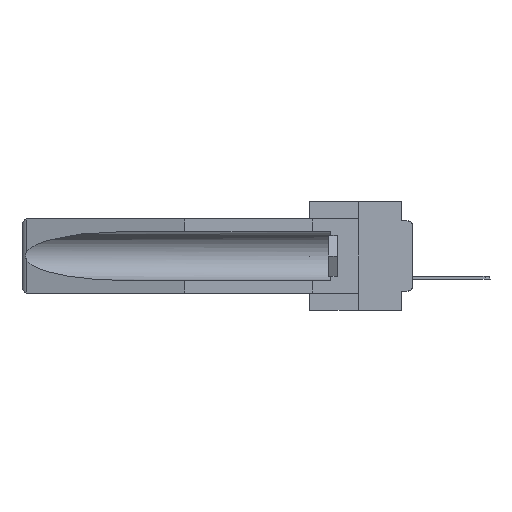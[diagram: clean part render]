
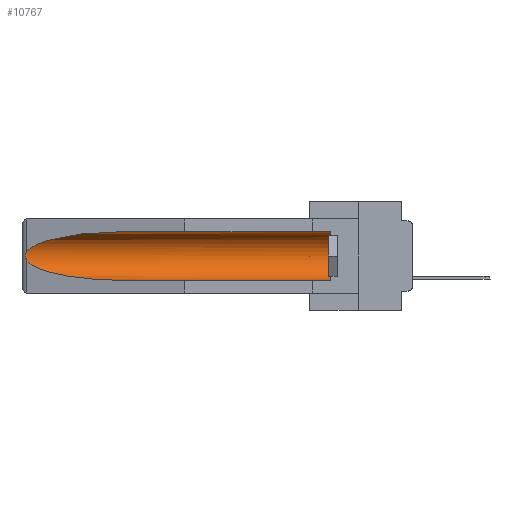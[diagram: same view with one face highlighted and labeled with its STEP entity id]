
A CAD part, left-side view. The second image highlights one B-rep face of the part: STEP entity #10767.
In plain terms, the highlighted cylindrical face has radius 2.857 mm (diameter 5.715 mm), a partial arc.
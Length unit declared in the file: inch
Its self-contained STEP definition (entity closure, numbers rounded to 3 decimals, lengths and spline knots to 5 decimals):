
#96 = ORIENTED_EDGE ( 'NONE', *, *, #34960, .F. ) ;
#110 = CARTESIAN_POINT ( 'NONE',  ( 0.25451, 1.48313, -0.09465 ) ) ;
#827 = CARTESIAN_POINT ( 'NONE',  ( 0.2673, 1.53269, -0.17917 ) ) ;
#1669 = VERTEX_POINT ( 'NONE', #9027 ) ;
#2537 = EDGE_CURVE ( 'NONE', #20760, #1669, #23115, .T. ) ;
#2706 = CARTESIAN_POINT ( 'NONE',  ( 0.155, -0.30754, -0.1715 ) ) ;
#2724 = CARTESIAN_POINT ( 'NONE',  ( 0.21114, 1.30732, -0.284 ) ) ;
#2728 = DIRECTION ( 'NONE',  ( 0., 1., 0. ) ) ;
#4487 = CARTESIAN_POINT ( 'NONE',  ( 0.26655, 1.53094, -0.18657 ) ) ;
#4593 = LINE ( 'NONE', #16008, #13410 ) ;
#5051 = B_SPLINE_CURVE_WITH_KNOTS ( 'NONE', 3,
 ( #12749, #19198, #12609, #27649, #9901, #18641, #827, #4487, #19465, #10458 ),
 .UNSPECIFIED., .F., .F.,
 ( 4, 2, 2, 2, 4 ),
 ( 0., 0.00029, 0.00058, 0.00087, 0.00117 ),
 .UNSPECIFIED. ) ;
#6569 = EDGE_CURVE ( 'NONE', #15668, #6992, #25724, .T. ) ;
#6992 = VERTEX_POINT ( 'NONE', #28050 ) ;
#7362 = CARTESIAN_POINT ( 'NONE',  ( 0.155, -0.30754, -0.059 ) ) ;
#7677 = VERTEX_POINT ( 'NONE', #29914 ) ;
#8663 = DIRECTION ( 'NONE',  ( 0., 0., 1. ) ) ;
#8772 = DIRECTION ( 'NONE',  ( 0., 1., 0. ) ) ;
#8886 = LINE ( 'NONE', #7362, #9338 ) ;
#9027 = CARTESIAN_POINT ( 'NONE',  ( 0.155, 0.126, -0.059 ) ) ;
#9338 = VECTOR ( 'NONE', #2728, 39.37008 ) ;
#9855 = EDGE_CURVE ( 'NONE', #1669, #15668, #8886, .T. ) ;
#9901 = CARTESIAN_POINT ( 'NONE',  ( 0.2675, 1.53308, -0.16763 ) ) ;
#10092 = ORIENTED_EDGE ( 'NONE', *, *, #10368, .T. ) ;
#10368 = EDGE_CURVE ( 'NONE', #7677, #26280, #29241, .T. ) ;
#10458 = CARTESIAN_POINT ( 'NONE',  ( 0.26537, 1.52718, -0.19328 ) ) ;
#10767 = ADVANCED_FACE ( 'NONE', ( #35269 ), #16749, .F. ) ;
#10997 = ORIENTED_EDGE ( 'NONE', *, *, #2537, .T. ) ;
#12609 = CARTESIAN_POINT ( 'NONE',  ( 0.26654, 1.53092, -0.15636 ) ) ;
#12749 = CARTESIAN_POINT ( 'NONE',  ( 0.26537, 1.52718, -0.14972 ) ) ;
#13410 = VECTOR ( 'NONE', #28172, 39.37008 ) ;
#14145 = CARTESIAN_POINT ( 'NONE',  ( 0.155, 1.07973, -0.059 ) ) ;
#14402 = CARTESIAN_POINT ( 'NONE',  ( 0.155, 1.07973, -0.059 ) ) ;
#15668 = VERTEX_POINT ( 'NONE', #14145 ) ;
#16008 = CARTESIAN_POINT ( 'NONE',  ( 0.155, -0.30754, -0.284 ) ) ;
#16749 = CYLINDRICAL_SURFACE ( 'NONE', #21634, 0.1125 ) ;
#17204 = EDGE_CURVE ( 'NONE', #6992, #7677, #5051, .T. ) ;
#18537 = CARTESIAN_POINT ( 'NONE',  ( 0.155, 1.07973, -0.284 ) ) ;
#18578 = CARTESIAN_POINT ( 'NONE',  ( 0.155, 0.126, -0.284 ) ) ;
#18641 = CARTESIAN_POINT ( 'NONE',  ( 0.2675, 1.53308, -0.17534 ) ) ;
#19198 = CARTESIAN_POINT ( 'NONE',  ( 0.26597, 1.52961, -0.15275 ) ) ;
#19465 = CARTESIAN_POINT ( 'NONE',  ( 0.26597, 1.5296, -0.19026 ) ) ;
#20276 = ORIENTED_EDGE ( 'NONE', *, *, #6569, .T. ) ;
#20760 = VERTEX_POINT ( 'NONE', #18578 ) ;
#21021 = ORIENTED_EDGE ( 'NONE', *, *, #9855, .T. ) ;
#21277 = DIRECTION ( 'NONE',  ( 0., 0., 1. ) ) ;
#21521 = EDGE_LOOP ( 'NONE', ( #20276, #30563, #10092, #96, #10997, #21021 ) ) ;
#21634 = AXIS2_PLACEMENT_3D ( 'NONE', #2706, #8772, #8663 ) ;
#23115 = CIRCLE ( 'NONE', #30518, 0.1125 ) ;
#23999 = DIRECTION ( 'NONE',  ( 0., -1., 0. ) ) ;
#25724 =( BOUNDED_CURVE ( )  B_SPLINE_CURVE ( 3, ( #14402, #38117, #110, #35527 ),
 .UNSPECIFIED., .F., .F. ) 
 B_SPLINE_CURVE_WITH_KNOTS ( ( 4, 4 ),
 ( 4.71239, 6.08839 ),
 .UNSPECIFIED. ) 
 CURVE ( )  GEOMETRIC_REPRESENTATION_ITEM ( )  RATIONAL_B_SPLINE_CURVE ( ( 1., 0.848, 0.848, 1. ) ) 
 REPRESENTATION_ITEM ( '' )  );
#26280 = VERTEX_POINT ( 'NONE', #18537 ) ;
#26774 = CARTESIAN_POINT ( 'NONE',  ( 0.155, 1.07973, -0.284 ) ) ;
#26827 = CARTESIAN_POINT ( 'NONE',  ( 0.155, 0.126, -0.1715 ) ) ;
#27649 = CARTESIAN_POINT ( 'NONE',  ( 0.2673, 1.5327, -0.16383 ) ) ;
#28050 = CARTESIAN_POINT ( 'NONE',  ( 0.26537, 1.52718, -0.14972 ) ) ;
#28172 = DIRECTION ( 'NONE',  ( 0., 1., 0. ) ) ;
#29241 =( BOUNDED_CURVE ( )  B_SPLINE_CURVE ( 3, ( #31758, #38086, #2724, #26774 ),
 .UNSPECIFIED., .F., .F. ) 
 B_SPLINE_CURVE_WITH_KNOTS ( ( 4, 4 ),
 ( 0.1948, 1.5708 ),
 .UNSPECIFIED. ) 
 CURVE ( )  GEOMETRIC_REPRESENTATION_ITEM ( )  RATIONAL_B_SPLINE_CURVE ( ( 1., 0.848, 0.848, 1. ) ) 
 REPRESENTATION_ITEM ( '' )  );
#29914 = CARTESIAN_POINT ( 'NONE',  ( 0.26537, 1.52718, -0.19328 ) ) ;
#30518 = AXIS2_PLACEMENT_3D ( 'NONE', #26827, #23999, #21277 ) ;
#30563 = ORIENTED_EDGE ( 'NONE', *, *, #17204, .T. ) ;
#31758 = CARTESIAN_POINT ( 'NONE',  ( 0.26537, 1.52718, -0.19328 ) ) ;
#34960 = EDGE_CURVE ( 'NONE', #20760, #26280, #4593, .T. ) ;
#35269 = FACE_OUTER_BOUND ( 'NONE', #21521, .T. ) ;
#35527 = CARTESIAN_POINT ( 'NONE',  ( 0.26537, 1.52718, -0.14972 ) ) ;
#38086 = CARTESIAN_POINT ( 'NONE',  ( 0.25451, 1.48313, -0.24835 ) ) ;
#38117 = CARTESIAN_POINT ( 'NONE',  ( 0.21114, 1.30732, -0.059 ) ) ;
